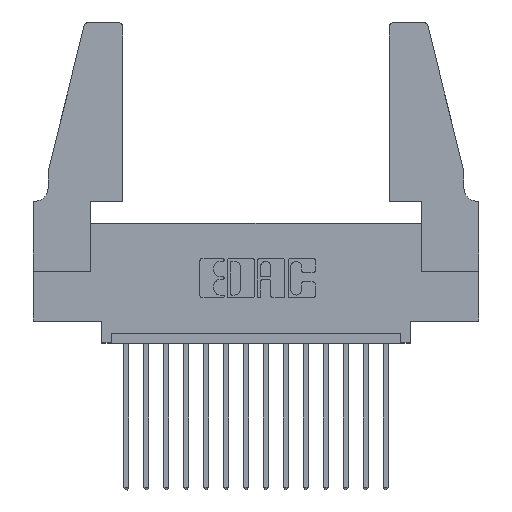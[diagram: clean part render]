
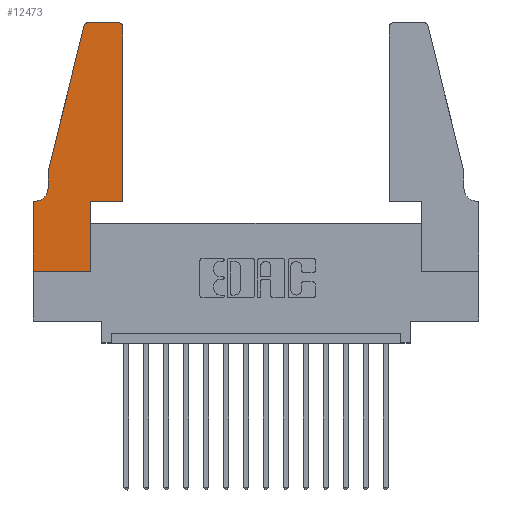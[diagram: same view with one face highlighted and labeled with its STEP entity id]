
A CAD part, top view. The second image highlights one B-rep face of the part: STEP entity #12473.
In plain terms, the highlighted planar face has unit normal (0, 0, 1).
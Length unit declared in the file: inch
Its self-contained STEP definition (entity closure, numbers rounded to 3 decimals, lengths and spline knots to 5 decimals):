
#100 = CARTESIAN_POINT ( 'NONE',  ( 0.2865, 0., 0.37 ) ) ;
#465 = ORIENTED_EDGE ( 'NONE', *, *, #3672, .T. ) ;
#807 = VERTEX_POINT ( 'NONE', #7876 ) ;
#835 = VERTEX_POINT ( 'NONE', #1302 ) ;
#861 = DIRECTION ( 'NONE',  ( 1., 0., 0. ) ) ;
#1302 = CARTESIAN_POINT ( 'NONE',  ( 0., 0.35, 0.37 ) ) ;
#1919 = CARTESIAN_POINT ( 'NONE',  ( 0.0055, 0.35, 0.37 ) ) ;
#2245 = ORIENTED_EDGE ( 'NONE', *, *, #14559, .T. ) ;
#2256 = PLANE ( 'NONE',  #16070 ) ;
#2286 = CARTESIAN_POINT ( 'NONE',  ( 0.4205, 1.22, 0.37 ) ) ;
#2573 = VERTEX_POINT ( 'NONE', #12727 ) ;
#2624 = VERTEX_POINT ( 'NONE', #6388 ) ;
#2745 = ORIENTED_EDGE ( 'NONE', *, *, #11406, .T. ) ;
#3095 = CARTESIAN_POINT ( 'NONE',  ( 0., 0., 0.37 ) ) ;
#3152 = EDGE_CURVE ( 'NONE', #835, #4851, #11581, .T. ) ;
#3601 = VERTEX_POINT ( 'NONE', #16020 ) ;
#3672 = EDGE_CURVE ( 'NONE', #2624, #6378, #4135, .T. ) ;
#3885 = CARTESIAN_POINT ( 'NONE',  ( 0.0755, 0.42, 0.37 ) ) ;
#4135 = LINE ( 'NONE', #16296, #7567 ) ;
#4422 = VECTOR ( 'NONE', #14446, 39.37008 ) ;
#4493 = CARTESIAN_POINT ( 'NONE',  ( 0.2865, 0.35, 0.37 ) ) ;
#4535 = CARTESIAN_POINT ( 'NONE',  ( 0., 0., 0.37 ) ) ;
#4656 = CARTESIAN_POINT ( 'NONE',  ( 0.4505, 1.22, 0.37 ) ) ;
#4851 = VERTEX_POINT ( 'NONE', #3095 ) ;
#4936 = VECTOR ( 'NONE', #11276, 39.37008 ) ;
#4957 = EDGE_CURVE ( 'NONE', #9965, #2573, #12746, .T. ) ;
#4994 = DIRECTION ( 'NONE',  ( -1., 0., 0. ) ) ;
#5437 = EDGE_CURVE ( 'NONE', #2573, #2624, #15931, .T. ) ;
#5654 = LINE ( 'NONE', #10181, #11699 ) ;
#5780 = VERTEX_POINT ( 'NONE', #1919 ) ;
#5804 = DIRECTION ( 'NONE',  ( 0., 1., 0. ) ) ;
#5963 = ORIENTED_EDGE ( 'NONE', *, *, #5437, .T. ) ;
#6002 = DIRECTION ( 'NONE',  ( 0., 0., 1. ) ) ;
#6005 = CARTESIAN_POINT ( 'NONE',  ( 0., 0., 0.37 ) ) ;
#6200 = DIRECTION ( 'NONE',  ( 0., 0., 1. ) ) ;
#6276 = ORIENTED_EDGE ( 'NONE', *, *, #13982, .T. ) ;
#6378 = VERTEX_POINT ( 'NONE', #4656 ) ;
#6388 = CARTESIAN_POINT ( 'NONE',  ( 0.4505, 0.35, 0.37 ) ) ;
#6722 = VECTOR ( 'NONE', #5804, 39.37008 ) ;
#6796 = ORIENTED_EDGE ( 'NONE', *, *, #13835, .T. ) ;
#6884 = VECTOR ( 'NONE', #9256, 39.37008 ) ;
#6902 = CIRCLE ( 'NONE', #9592, 0.03 ) ;
#7063 = CARTESIAN_POINT ( 'NONE',  ( 0.0755, 0.35, 0.37 ) ) ;
#7237 = DIRECTION ( 'NONE',  ( 0., 0., 1. ) ) ;
#7291 = DIRECTION ( 'NONE',  ( 1., 0., 0. ) ) ;
#7567 = VECTOR ( 'NONE', #11117, 39.37008 ) ;
#7876 = CARTESIAN_POINT ( 'NONE',  ( 0.284, 1.25, 0.37 ) ) ;
#8807 = DIRECTION ( 'NONE',  ( 0., -1., 0. ) ) ;
#9010 = VECTOR ( 'NONE', #8807, 39.37008 ) ;
#9063 = LINE ( 'NONE', #15690, #4422 ) ;
#9072 = DIRECTION ( 'NONE',  ( 0., 0., -1. ) ) ;
#9085 = ORIENTED_EDGE ( 'NONE', *, *, #10902, .T. ) ;
#9127 = DIRECTION ( 'NONE',  ( -1., 0., 0. ) ) ;
#9256 = DIRECTION ( 'NONE',  ( 1., 0., 0. ) ) ;
#9478 = ORIENTED_EDGE ( 'NONE', *, *, #13909, .T. ) ;
#9592 = AXIS2_PLACEMENT_3D ( 'NONE', #2286, #6200, #13790 ) ;
#9717 = CARTESIAN_POINT ( 'NONE',  ( 0.284, 1.22, 0.37 ) ) ;
#9965 = VERTEX_POINT ( 'NONE', #100 ) ;
#9996 = CARTESIAN_POINT ( 'NONE',  ( 0., 0.35, 0.37 ) ) ;
#10181 = CARTESIAN_POINT ( 'NONE',  ( 0.2605, 1.25, 0.37 ) ) ;
#10419 = LINE ( 'NONE', #12606, #9010 ) ;
#10490 = AXIS2_PLACEMENT_3D ( 'NONE', #14194, #9072, #9127 ) ;
#10501 = CIRCLE ( 'NONE', #10490, 0.07 ) ;
#10831 = ORIENTED_EDGE ( 'NONE', *, *, #3152, .T. ) ;
#10902 = EDGE_CURVE ( 'NONE', #807, #11684, #14984, .T. ) ;
#10919 = CARTESIAN_POINT ( 'NONE',  ( 0.25487, 1.22718, 0.37 ) ) ;
#11108 = DIRECTION ( 'NONE',  ( 1., 0., 0. ) ) ;
#11117 = DIRECTION ( 'NONE',  ( 0., 1., 0. ) ) ;
#11276 = DIRECTION ( 'NONE',  ( 0., -1., 0. ) ) ;
#11406 = EDGE_CURVE ( 'NONE', #6378, #16200, #6902, .T. ) ;
#11581 = LINE ( 'NONE', #4535, #4936 ) ;
#11684 = VERTEX_POINT ( 'NONE', #10919 ) ;
#11699 = VECTOR ( 'NONE', #4994, 39.37008 ) ;
#11783 = CARTESIAN_POINT ( 'NONE',  ( 0.4505, 0.35, 0.37 ) ) ;
#12319 = VERTEX_POINT ( 'NONE', #3885 ) ;
#12337 = FACE_OUTER_BOUND ( 'NONE', #13520, .T. ) ;
#12473 = ADVANCED_FACE ( 'NONE', ( #12337 ), #2256, .T. ) ;
#12606 = CARTESIAN_POINT ( 'NONE',  ( 0.0755, 0.5, 0.37 ) ) ;
#12657 = ORIENTED_EDGE ( 'NONE', *, *, #15469, .T. ) ;
#12660 = ORIENTED_EDGE ( 'NONE', *, *, #4957, .T. ) ;
#12727 = CARTESIAN_POINT ( 'NONE',  ( 0.2865, 0.35, 0.37 ) ) ;
#12746 = LINE ( 'NONE', #4493, #6722 ) ;
#13148 = AXIS2_PLACEMENT_3D ( 'NONE', #9717, #7237, #861 ) ;
#13520 = EDGE_LOOP ( 'NONE', ( #6276, #9085, #15972, #12657, #9478, #2245, #10831, #6796, #12660, #5963, #465, #2745 ) ) ;
#13790 = DIRECTION ( 'NONE',  ( 1., 0., 0. ) ) ;
#13835 = EDGE_CURVE ( 'NONE', #4851, #9965, #14325, .T. ) ;
#13909 = EDGE_CURVE ( 'NONE', #12319, #5780, #10501, .T. ) ;
#13982 = EDGE_CURVE ( 'NONE', #16200, #807, #5654, .T. ) ;
#14194 = CARTESIAN_POINT ( 'NONE',  ( 0.0055, 0.42, 0.37 ) ) ;
#14248 = EDGE_CURVE ( 'NONE', #11684, #3601, #9063, .T. ) ;
#14325 = LINE ( 'NONE', #6005, #15135 ) ;
#14446 = DIRECTION ( 'NONE',  ( -0.239, -0.971, 0. ) ) ;
#14559 = EDGE_CURVE ( 'NONE', #5780, #835, #14888, .T. ) ;
#14885 = DIRECTION ( 'NONE',  ( -1., 0., 0. ) ) ;
#14888 = LINE ( 'NONE', #7063, #16501 ) ;
#14984 = CIRCLE ( 'NONE', #13148, 0.03 ) ;
#15135 = VECTOR ( 'NONE', #11108, 39.37008 ) ;
#15246 = CARTESIAN_POINT ( 'NONE',  ( 0.4205, 1.25, 0.37 ) ) ;
#15469 = EDGE_CURVE ( 'NONE', #3601, #12319, #10419, .T. ) ;
#15690 = CARTESIAN_POINT ( 'NONE',  ( 0.0755, 0.5, 0.37 ) ) ;
#15931 = LINE ( 'NONE', #11783, #6884 ) ;
#15972 = ORIENTED_EDGE ( 'NONE', *, *, #14248, .T. ) ;
#16020 = CARTESIAN_POINT ( 'NONE',  ( 0.0755, 0.5, 0.37 ) ) ;
#16070 = AXIS2_PLACEMENT_3D ( 'NONE', #9996, #6002, #7291 ) ;
#16200 = VERTEX_POINT ( 'NONE', #15246 ) ;
#16296 = CARTESIAN_POINT ( 'NONE',  ( 0.4505, 0.35, 0.37 ) ) ;
#16501 = VECTOR ( 'NONE', #14885, 39.37008 ) ;
